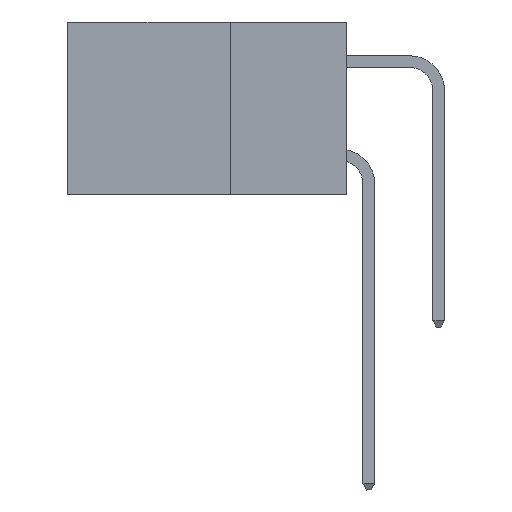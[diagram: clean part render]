
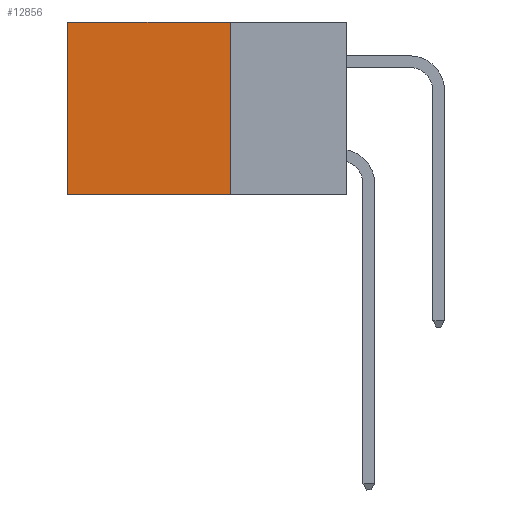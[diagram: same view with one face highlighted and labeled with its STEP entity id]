
A CAD part, left-side view. The second image highlights one B-rep face of the part: STEP entity #12856.
In plain terms, the highlighted planar face has unit normal (-1, 0, 0).
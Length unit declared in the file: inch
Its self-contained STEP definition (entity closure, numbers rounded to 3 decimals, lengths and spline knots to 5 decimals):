
#72 = CARTESIAN_POINT ( 'NONE',  ( 0.2875, 0.6, 0. ) ) ;
#1364 = ORIENTED_EDGE ( 'NONE', *, *, #9333, .T. ) ;
#2116 = ORIENTED_EDGE ( 'NONE', *, *, #2959, .T. ) ;
#2293 = CARTESIAN_POINT ( 'NONE',  ( 0.2875, 0.25, 0. ) ) ;
#2437 = VERTEX_POINT ( 'NONE', #15518 ) ;
#2959 = EDGE_CURVE ( 'NONE', #4933, #14359, #9881, .T. ) ;
#4338 = DIRECTION ( 'NONE',  ( 0., 1., 0. ) ) ;
#4346 = VECTOR ( 'NONE', #7097, 39.37008 ) ;
#4916 = DIRECTION ( 'NONE',  ( 0., 0., -1. ) ) ;
#4933 = VERTEX_POINT ( 'NONE', #72 ) ;
#5152 = VERTEX_POINT ( 'NONE', #9983 ) ;
#6312 = VECTOR ( 'NONE', #4916, 39.37008 ) ;
#6486 = VECTOR ( 'NONE', #21707, 39.37008 ) ;
#7097 = DIRECTION ( 'NONE',  ( 0., 0., -1. ) ) ;
#7364 = FACE_OUTER_BOUND ( 'NONE', #17831, .T. ) ;
#7673 = EDGE_CURVE ( 'NONE', #5152, #2437, #11262, .T. ) ;
#8557 = DIRECTION ( 'NONE',  ( 1., 0., 0. ) ) ;
#9141 = VECTOR ( 'NONE', #4338, 39.37008 ) ;
#9333 = EDGE_CURVE ( 'NONE', #5152, #4933, #23845, .T. ) ;
#9881 = LINE ( 'NONE', #10806, #4346 ) ;
#9983 = CARTESIAN_POINT ( 'NONE',  ( 0.2875, 0.25, 0. ) ) ;
#10806 = CARTESIAN_POINT ( 'NONE',  ( 0.2875, 0.6, 0. ) ) ;
#11103 = CARTESIAN_POINT ( 'NONE',  ( 0.2875, 0.6, -0.37 ) ) ;
#11262 = LINE ( 'NONE', #23354, #6312 ) ;
#12856 = ADVANCED_FACE ( 'NONE', ( #7364 ), #17806, .F. ) ;
#14359 = VERTEX_POINT ( 'NONE', #11103 ) ;
#15518 = CARTESIAN_POINT ( 'NONE',  ( 0.2875, 0.25, -0.37 ) ) ;
#16228 = CARTESIAN_POINT ( 'NONE',  ( 0.2875, 0.25, -0.37 ) ) ;
#16332 = LINE ( 'NONE', #16228, #6486 ) ;
#16902 = AXIS2_PLACEMENT_3D ( 'NONE', #19655, #8557, #21499 ) ;
#17806 = PLANE ( 'NONE',  #16902 ) ;
#17831 = EDGE_LOOP ( 'NONE', ( #2116, #19189, #21713, #1364 ) ) ;
#18046 = EDGE_CURVE ( 'NONE', #2437, #14359, #16332, .T. ) ;
#19189 = ORIENTED_EDGE ( 'NONE', *, *, #18046, .F. ) ;
#19655 = CARTESIAN_POINT ( 'NONE',  ( 0.2875, 0.25, 0. ) ) ;
#21499 = DIRECTION ( 'NONE',  ( 0., 0., -1. ) ) ;
#21707 = DIRECTION ( 'NONE',  ( 0., 1., 0. ) ) ;
#21713 = ORIENTED_EDGE ( 'NONE', *, *, #7673, .F. ) ;
#23354 = CARTESIAN_POINT ( 'NONE',  ( 0.2875, 0.25, 0. ) ) ;
#23845 = LINE ( 'NONE', #2293, #9141 ) ;
